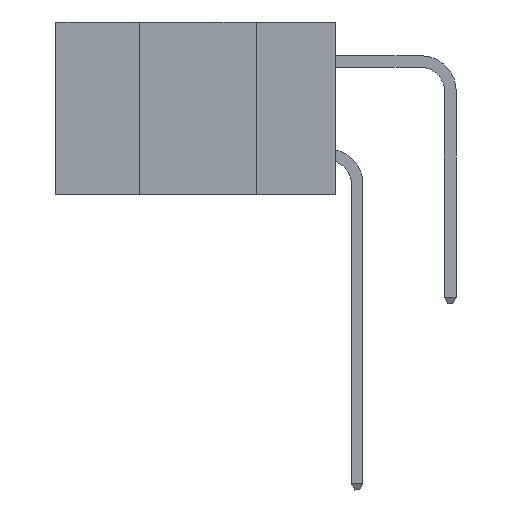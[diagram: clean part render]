
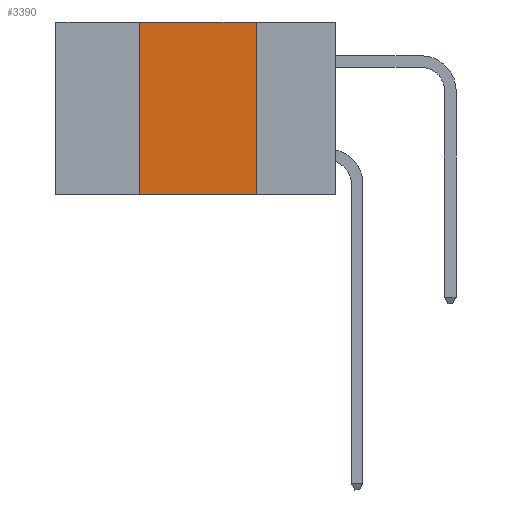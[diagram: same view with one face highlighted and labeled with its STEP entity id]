
A CAD part, left-side view. The second image highlights one B-rep face of the part: STEP entity #3390.
In plain terms, the highlighted planar face has unit normal (-1, 0, 0).
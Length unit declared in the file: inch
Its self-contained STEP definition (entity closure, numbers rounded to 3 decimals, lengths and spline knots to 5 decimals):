
#1051 = CARTESIAN_POINT ( 'NONE',  ( 0., 0.6, 0. ) ) ;
#1352 = DIRECTION ( 'NONE',  ( 0., 0., -1. ) ) ;
#1502 = CARTESIAN_POINT ( 'NONE',  ( 0., 0.42, 0. ) ) ;
#3051 = LINE ( 'NONE', #19638, #11680 ) ;
#3390 = ADVANCED_FACE ( 'NONE', ( #15522 ), #17459, .F. ) ;
#3458 = CARTESIAN_POINT ( 'NONE',  ( 0., 0.42, -0.37 ) ) ;
#4077 = VERTEX_POINT ( 'NONE', #11343 ) ;
#5959 = EDGE_CURVE ( 'NONE', #11372, #15017, #14178, .T. ) ;
#6097 = EDGE_CURVE ( 'NONE', #18944, #15017, #3051, .T. ) ;
#7883 = CARTESIAN_POINT ( 'NONE',  ( 0., 0.17, 0. ) ) ;
#7902 = DIRECTION ( 'NONE',  ( 0., 0., 1. ) ) ;
#8125 = DIRECTION ( 'NONE',  ( 0., 0., -1. ) ) ;
#8742 = EDGE_LOOP ( 'NONE', ( #12873, #12928, #13087, #13106 ) ) ;
#9512 = CARTESIAN_POINT ( 'NONE',  ( 0., 0.6, 0. ) ) ;
#10004 = DIRECTION ( 'NONE',  ( 0., -1., 0. ) ) ;
#10790 = EDGE_CURVE ( 'NONE', #18944, #4077, #12264, .T. ) ;
#10848 = DIRECTION ( 'NONE',  ( 0., -1., 0. ) ) ;
#11121 = DIRECTION ( 'NONE',  ( 1., 0., 0. ) ) ;
#11343 = CARTESIAN_POINT ( 'NONE',  ( 0., 0.42, 0. ) ) ;
#11372 = VERTEX_POINT ( 'NONE', #7883 ) ;
#11680 = VECTOR ( 'NONE', #10004, 39.37008 ) ;
#12264 = LINE ( 'NONE', #1502, #20273 ) ;
#12873 = ORIENTED_EDGE ( 'NONE', *, *, #5959, .F. ) ;
#12928 = ORIENTED_EDGE ( 'NONE', *, *, #17723, .F. ) ;
#13087 = ORIENTED_EDGE ( 'NONE', *, *, #10790, .F. ) ;
#13106 = ORIENTED_EDGE ( 'NONE', *, *, #6097, .T. ) ;
#13597 = AXIS2_PLACEMENT_3D ( 'NONE', #9512, #11121, #1352 ) ;
#14178 = LINE ( 'NONE', #14514, #17912 ) ;
#14405 = VECTOR ( 'NONE', #10848, 39.37008 ) ;
#14514 = CARTESIAN_POINT ( 'NONE',  ( 0., 0.17, 0. ) ) ;
#15017 = VERTEX_POINT ( 'NONE', #18210 ) ;
#15522 = FACE_OUTER_BOUND ( 'NONE', #8742, .T. ) ;
#17459 = PLANE ( 'NONE',  #13597 ) ;
#17723 = EDGE_CURVE ( 'NONE', #4077, #11372, #18139, .T. ) ;
#17912 = VECTOR ( 'NONE', #8125, 39.37008 ) ;
#18139 = LINE ( 'NONE', #1051, #14405 ) ;
#18210 = CARTESIAN_POINT ( 'NONE',  ( 0., 0.17, -0.37 ) ) ;
#18944 = VERTEX_POINT ( 'NONE', #3458 ) ;
#19638 = CARTESIAN_POINT ( 'NONE',  ( 0., 0.6, -0.37 ) ) ;
#20273 = VECTOR ( 'NONE', #7902, 39.37008 ) ;
